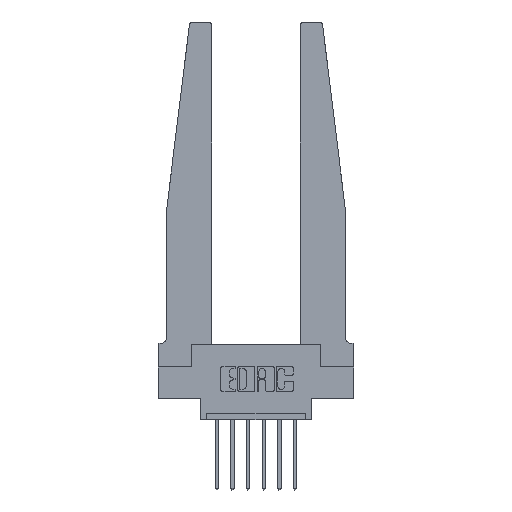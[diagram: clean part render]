
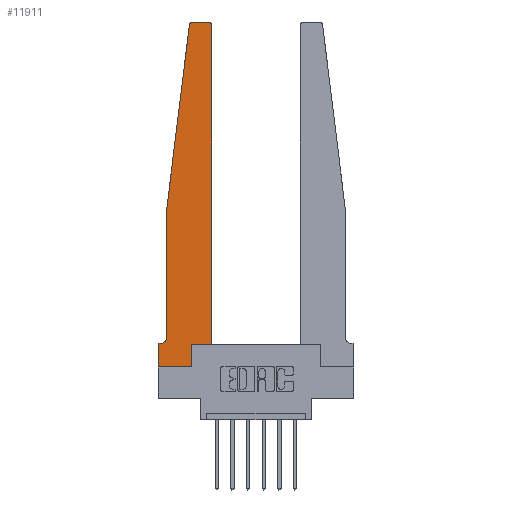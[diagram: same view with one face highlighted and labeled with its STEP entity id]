
A CAD part, top view. The second image highlights one B-rep face of the part: STEP entity #11911.
In plain terms, the highlighted planar face has unit normal (0, 0, 1).
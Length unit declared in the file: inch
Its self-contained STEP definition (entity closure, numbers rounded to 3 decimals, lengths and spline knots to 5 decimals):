
#217 = CIRCLE ( 'NONE', #8093, 0.03 ) ;
#237 = AXIS2_PLACEMENT_3D ( 'NONE', #9113, #8110, #11270 ) ;
#318 = VERTEX_POINT ( 'NONE', #1391 ) ;
#476 = ORIENTED_EDGE ( 'NONE', *, *, #4380, .T. ) ;
#621 = CARTESIAN_POINT ( 'NONE',  ( 0.2605, 0.18, 0.37 ) ) ;
#788 = AXIS2_PLACEMENT_3D ( 'NONE', #11460, #5144, #1828 ) ;
#809 = ORIENTED_EDGE ( 'NONE', *, *, #1120, .T. ) ;
#859 = VERTEX_POINT ( 'NONE', #12842 ) ;
#991 = DIRECTION ( 'NONE',  ( -0.122, -0.992, 0. ) ) ;
#1015 = AXIS2_PLACEMENT_3D ( 'NONE', #13551, #3934, #7163 ) ;
#1099 = LINE ( 'NONE', #7585, #3458 ) ;
#1120 = EDGE_CURVE ( 'NONE', #7941, #2557, #12150, .T. ) ;
#1167 = DIRECTION ( 'NONE',  ( -1., 0., 0. ) ) ;
#1228 = EDGE_CURVE ( 'NONE', #7506, #8497, #217, .T. ) ;
#1383 = EDGE_CURVE ( 'NONE', #8497, #7941, #4676, .T. ) ;
#1391 = CARTESIAN_POINT ( 'NONE',  ( 0.065, 0.2375, 0.37 ) ) ;
#1828 = DIRECTION ( 'NONE',  ( -1., 0., 0. ) ) ;
#1990 = CARTESIAN_POINT ( 'NONE',  ( 0.065, 1.25, 0.37 ) ) ;
#2323 = VECTOR ( 'NONE', #3378, 39.37008 ) ;
#2425 = ORIENTED_EDGE ( 'NONE', *, *, #10086, .T. ) ;
#2480 = VECTOR ( 'NONE', #7611, 39.37008 ) ;
#2557 = VERTEX_POINT ( 'NONE', #9505 ) ;
#2607 = VECTOR ( 'NONE', #6348, 39.37008 ) ;
#2664 = ORIENTED_EDGE ( 'NONE', *, *, #1383, .T. ) ;
#2727 = CARTESIAN_POINT ( 'NONE',  ( 0.2605, 0.18, 0.37 ) ) ;
#2945 = ORIENTED_EDGE ( 'NONE', *, *, #12393, .T. ) ;
#3117 = CARTESIAN_POINT ( 'NONE',  ( 0., 0., 0.37 ) ) ;
#3323 = LINE ( 'NONE', #6544, #2480 ) ;
#3378 = DIRECTION ( 'NONE',  ( 1., 0., 0. ) ) ;
#3458 = VECTOR ( 'NONE', #1167, 39.37008 ) ;
#3798 = LINE ( 'NONE', #13484, #4347 ) ;
#3934 = DIRECTION ( 'NONE',  ( 0., 0., 1. ) ) ;
#4138 = LINE ( 'NONE', #6210, #8124 ) ;
#4211 = CARTESIAN_POINT ( 'NONE',  ( 0.425, 2.72, 0.37 ) ) ;
#4347 = VECTOR ( 'NONE', #9961, 39.37008 ) ;
#4380 = EDGE_CURVE ( 'NONE', #318, #12587, #9999, .T. ) ;
#4644 = ORIENTED_EDGE ( 'NONE', *, *, #8417, .T. ) ;
#4676 = LINE ( 'NONE', #8955, #5438 ) ;
#5144 = DIRECTION ( 'NONE',  ( 0., 0., -1. ) ) ;
#5326 = ORIENTED_EDGE ( 'NONE', *, *, #12911, .T. ) ;
#5404 = EDGE_CURVE ( 'NONE', #859, #7506, #3323, .T. ) ;
#5438 = VECTOR ( 'NONE', #13236, 39.37008 ) ;
#6162 = EDGE_CURVE ( 'NONE', #6501, #7815, #3798, .T. ) ;
#6206 = LINE ( 'NONE', #11571, #2607 ) ;
#6210 = CARTESIAN_POINT ( 'NONE',  ( 0.065, 1.25, 0.37 ) ) ;
#6312 = CARTESIAN_POINT ( 'NONE',  ( 0.2605, 0., 0.37 ) ) ;
#6348 = DIRECTION ( 'NONE',  ( 1., 0., 0. ) ) ;
#6435 = EDGE_CURVE ( 'NONE', #12980, #318, #4138, .T. ) ;
#6501 = VERTEX_POINT ( 'NONE', #9794 ) ;
#6544 = CARTESIAN_POINT ( 'NONE',  ( 0.425, 0.18, 0.37 ) ) ;
#6633 = EDGE_LOOP ( 'NONE', ( #2664, #809, #5326, #13695, #476, #2425, #10019, #2945, #9824, #4644, #10239, #12132 ) ) ;
#6671 = CARTESIAN_POINT ( 'NONE',  ( 0.425, 0.18, 0.37 ) ) ;
#6815 = CARTESIAN_POINT ( 'NONE',  ( 0.395, 2.75, 0.37 ) ) ;
#7163 = DIRECTION ( 'NONE',  ( 1., 0., 0. ) ) ;
#7506 = VERTEX_POINT ( 'NONE', #4211 ) ;
#7585 = CARTESIAN_POINT ( 'NONE',  ( 0.065, 0.1875, 0.37 ) ) ;
#7611 = DIRECTION ( 'NONE',  ( 0., 1., 0. ) ) ;
#7815 = VERTEX_POINT ( 'NONE', #3117 ) ;
#7941 = VERTEX_POINT ( 'NONE', #9909 ) ;
#8093 = AXIS2_PLACEMENT_3D ( 'NONE', #9592, #8543, #11775 ) ;
#8110 = DIRECTION ( 'NONE',  ( 0., 0., 1. ) ) ;
#8124 = VECTOR ( 'NONE', #10926, 39.37008 ) ;
#8145 = LINE ( 'NONE', #621, #8640 ) ;
#8417 = EDGE_CURVE ( 'NONE', #10553, #859, #13011, .T. ) ;
#8497 = VERTEX_POINT ( 'NONE', #6815 ) ;
#8543 = DIRECTION ( 'NONE',  ( 0., 0., 1. ) ) ;
#8640 = VECTOR ( 'NONE', #11598, 39.37008 ) ;
#8955 = CARTESIAN_POINT ( 'NONE',  ( 0.25, 2.75, 0.37 ) ) ;
#9113 = CARTESIAN_POINT ( 'NONE',  ( 0.27653, 2.72, 0.37 ) ) ;
#9505 = CARTESIAN_POINT ( 'NONE',  ( 0.24675, 2.72367, 0.37 ) ) ;
#9592 = CARTESIAN_POINT ( 'NONE',  ( 0.395, 2.72, 0.37 ) ) ;
#9794 = CARTESIAN_POINT ( 'NONE',  ( 0., 0.1875, 0.37 ) ) ;
#9824 = ORIENTED_EDGE ( 'NONE', *, *, #10565, .T. ) ;
#9909 = CARTESIAN_POINT ( 'NONE',  ( 0.27653, 2.75, 0.37 ) ) ;
#9961 = DIRECTION ( 'NONE',  ( 0., -1., 0. ) ) ;
#9999 = CIRCLE ( 'NONE', #788, 0.05 ) ;
#10019 = ORIENTED_EDGE ( 'NONE', *, *, #6162, .T. ) ;
#10086 = EDGE_CURVE ( 'NONE', #12587, #6501, #1099, .T. ) ;
#10239 = ORIENTED_EDGE ( 'NONE', *, *, #5404, .T. ) ;
#10553 = VERTEX_POINT ( 'NONE', #2727 ) ;
#10565 = EDGE_CURVE ( 'NONE', #13327, #10553, #8145, .T. ) ;
#10627 = LINE ( 'NONE', #1990, #12957 ) ;
#10926 = DIRECTION ( 'NONE',  ( 0., -1., 0. ) ) ;
#11106 = FACE_OUTER_BOUND ( 'NONE', #6633, .T. ) ;
#11270 = DIRECTION ( 'NONE',  ( 1., 0., 0. ) ) ;
#11367 = PLANE ( 'NONE',  #1015 ) ;
#11460 = CARTESIAN_POINT ( 'NONE',  ( 0.015, 0.2375, 0.37 ) ) ;
#11571 = CARTESIAN_POINT ( 'NONE',  ( 0., 0., 0.37 ) ) ;
#11598 = DIRECTION ( 'NONE',  ( 0., 1., 0. ) ) ;
#11775 = DIRECTION ( 'NONE',  ( 1., 0., 0. ) ) ;
#11911 = ADVANCED_FACE ( 'NONE', ( #11106 ), #11367, .T. ) ;
#12132 = ORIENTED_EDGE ( 'NONE', *, *, #1228, .T. ) ;
#12150 = CIRCLE ( 'NONE', #237, 0.03 ) ;
#12198 = CARTESIAN_POINT ( 'NONE',  ( 0.015, 0.1875, 0.37 ) ) ;
#12393 = EDGE_CURVE ( 'NONE', #7815, #13327, #6206, .T. ) ;
#12587 = VERTEX_POINT ( 'NONE', #12198 ) ;
#12842 = CARTESIAN_POINT ( 'NONE',  ( 0.425, 0.18, 0.37 ) ) ;
#12911 = EDGE_CURVE ( 'NONE', #2557, #12980, #10627, .T. ) ;
#12957 = VECTOR ( 'NONE', #991, 39.37008 ) ;
#12980 = VERTEX_POINT ( 'NONE', #13806 ) ;
#13011 = LINE ( 'NONE', #6671, #2323 ) ;
#13236 = DIRECTION ( 'NONE',  ( -1., 0., 0. ) ) ;
#13327 = VERTEX_POINT ( 'NONE', #6312 ) ;
#13484 = CARTESIAN_POINT ( 'NONE',  ( 0., 0., 0.37 ) ) ;
#13551 = CARTESIAN_POINT ( 'NONE',  ( 0., 0.1875, 0.37 ) ) ;
#13695 = ORIENTED_EDGE ( 'NONE', *, *, #6435, .T. ) ;
#13806 = CARTESIAN_POINT ( 'NONE',  ( 0.065, 1.25, 0.37 ) ) ;
